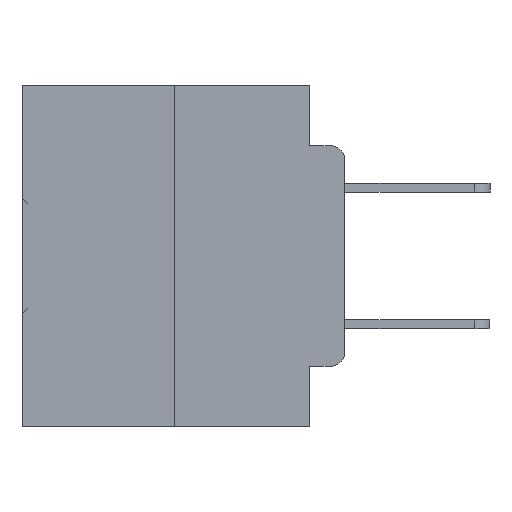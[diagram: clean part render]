
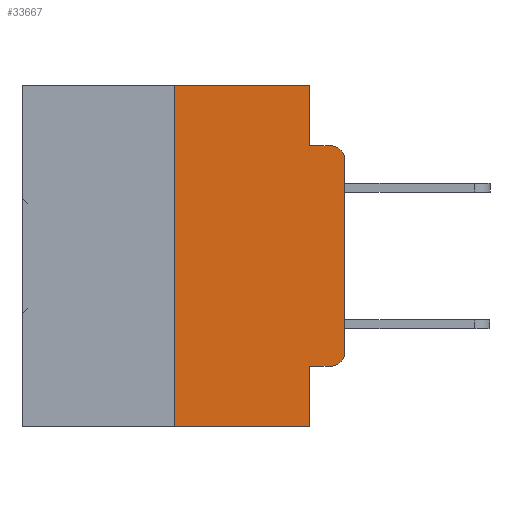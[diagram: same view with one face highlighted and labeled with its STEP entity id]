
A CAD part, left-side view. The second image highlights one B-rep face of the part: STEP entity #33667.
In plain terms, the highlighted planar face has unit normal (-1, 0, 0).
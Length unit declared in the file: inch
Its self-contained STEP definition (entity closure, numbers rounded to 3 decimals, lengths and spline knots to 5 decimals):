
#145 = EDGE_CURVE ( 'NONE', #18200, #20704, #22576, .T. ) ;
#853 = DIRECTION ( 'NONE',  ( 0., -1., 0. ) ) ;
#1075 = DIRECTION ( 'NONE',  ( 0., 0., -1. ) ) ;
#1307 = VERTEX_POINT ( 'NONE', #23346 ) ;
#1445 = CARTESIAN_POINT ( 'NONE',  ( 0., 0.051, 0. ) ) ;
#1585 = DIRECTION ( 'NONE',  ( 0., 0., -1. ) ) ;
#1717 = ORIENTED_EDGE ( 'NONE', *, *, #8641, .T. ) ;
#2132 = EDGE_CURVE ( 'NONE', #2736, #20704, #12573, .T. ) ;
#2736 = VERTEX_POINT ( 'NONE', #16717 ) ;
#3156 = DIRECTION ( 'NONE',  ( -1., 0., 0. ) ) ;
#4194 = DIRECTION ( 'NONE',  ( 0., -1., 0. ) ) ;
#4334 = ORIENTED_EDGE ( 'NONE', *, *, #32580, .T. ) ;
#4519 = PLANE ( 'NONE',  #10780 ) ;
#4811 = EDGE_CURVE ( 'NONE', #11716, #18200, #18731, .T. ) ;
#5305 = VERTEX_POINT ( 'NONE', #17956 ) ;
#5535 = VERTEX_POINT ( 'NONE', #29297 ) ;
#5775 = VECTOR ( 'NONE', #8782, 39.37008 ) ;
#7265 = CARTESIAN_POINT ( 'NONE',  ( 0., 0.473, 0. ) ) ;
#7304 = VERTEX_POINT ( 'NONE', #12982 ) ;
#7337 = LINE ( 'NONE', #9028, #33947 ) ;
#7715 = ORIENTED_EDGE ( 'NONE', *, *, #4811, .T. ) ;
#7801 = CARTESIAN_POINT ( 'NONE',  ( 0., 0.02, -0.4115 ) ) ;
#7810 = ORIENTED_EDGE ( 'NONE', *, *, #27281, .F. ) ;
#8641 = EDGE_CURVE ( 'NONE', #1307, #5305, #13774, .T. ) ;
#8782 = DIRECTION ( 'NONE',  ( 0., -1., 0. ) ) ;
#9028 = CARTESIAN_POINT ( 'NONE',  ( 0., 0.473, 0. ) ) ;
#9862 = AXIS2_PLACEMENT_3D ( 'NONE', #19339, #3156, #22029 ) ;
#10780 = AXIS2_PLACEMENT_3D ( 'NONE', #7265, #12646, #31262 ) ;
#11015 = AXIS2_PLACEMENT_3D ( 'NONE', #27876, #27852, #1075 ) ;
#11169 = CARTESIAN_POINT ( 'NONE',  ( 0., 0., -0.3915 ) ) ;
#11379 = CARTESIAN_POINT ( 'NONE',  ( 0., 0.25, 0. ) ) ;
#11716 = VERTEX_POINT ( 'NONE', #11169 ) ;
#11877 = VECTOR ( 'NONE', #853, 39.37008 ) ;
#12272 = EDGE_CURVE ( 'NONE', #1307, #7304, #22012, .T. ) ;
#12573 = LINE ( 'NONE', #17538, #26026 ) ;
#12646 = DIRECTION ( 'NONE',  ( 1., 0., 0. ) ) ;
#12814 = ORIENTED_EDGE ( 'NONE', *, *, #2132, .F. ) ;
#12982 = CARTESIAN_POINT ( 'NONE',  ( 0., 0.25, 0. ) ) ;
#13774 = LINE ( 'NONE', #27489, #5775 ) ;
#15287 = ORIENTED_EDGE ( 'NONE', *, *, #17733, .T. ) ;
#15960 = EDGE_LOOP ( 'NONE', ( #7715, #29438, #12814, #7810, #26127, #20745, #1717, #34269, #15287, #4334 ) ) ;
#16717 = CARTESIAN_POINT ( 'NONE',  ( 0., 0.051, -0.0885 ) ) ;
#17164 = DIRECTION ( 'NONE',  ( 0., -1., 0. ) ) ;
#17538 = CARTESIAN_POINT ( 'NONE',  ( 0., 0.051, -0.0885 ) ) ;
#17641 = DIRECTION ( 'NONE',  ( 0., 0., -1. ) ) ;
#17733 = EDGE_CURVE ( 'NONE', #26910, #34404, #19081, .T. ) ;
#17956 = CARTESIAN_POINT ( 'NONE',  ( 0., 0.051, -0.5 ) ) ;
#18200 = VERTEX_POINT ( 'NONE', #29771 ) ;
#18731 = LINE ( 'NONE', #21404, #26636 ) ;
#18932 = VECTOR ( 'NONE', #17641, 39.37008 ) ;
#19081 = LINE ( 'NONE', #19543, #11877 ) ;
#19339 = CARTESIAN_POINT ( 'NONE',  ( 0., 0.02, -0.3915 ) ) ;
#19543 = CARTESIAN_POINT ( 'NONE',  ( 0., 0.051, -0.4115 ) ) ;
#19749 = FACE_OUTER_BOUND ( 'NONE', #15960, .T. ) ;
#20349 = VECTOR ( 'NONE', #22112, 39.37008 ) ;
#20682 = EDGE_CURVE ( 'NONE', #26910, #5305, #34568, .T. ) ;
#20704 = VERTEX_POINT ( 'NONE', #31043 ) ;
#20745 = ORIENTED_EDGE ( 'NONE', *, *, #12272, .F. ) ;
#21404 = CARTESIAN_POINT ( 'NONE',  ( 0., 0., 0. ) ) ;
#21786 = CARTESIAN_POINT ( 'NONE',  ( 0., 0.051, -0.4115 ) ) ;
#22012 = LINE ( 'NONE', #11379, #20349 ) ;
#22029 = DIRECTION ( 'NONE',  ( 0., 0., -1. ) ) ;
#22112 = DIRECTION ( 'NONE',  ( 0., 0., 1. ) ) ;
#22388 = VECTOR ( 'NONE', #1585, 39.37008 ) ;
#22576 = CIRCLE ( 'NONE', #11015, 0.02 ) ;
#23346 = CARTESIAN_POINT ( 'NONE',  ( 0., 0.25, -0.5 ) ) ;
#24081 = DIRECTION ( 'NONE',  ( 0., 0., 1. ) ) ;
#26026 = VECTOR ( 'NONE', #4194, 39.37008 ) ;
#26127 = ORIENTED_EDGE ( 'NONE', *, *, #31500, .F. ) ;
#26636 = VECTOR ( 'NONE', #24081, 39.37008 ) ;
#26827 = CIRCLE ( 'NONE', #9862, 0.02 ) ;
#26910 = VERTEX_POINT ( 'NONE', #21786 ) ;
#27281 = EDGE_CURVE ( 'NONE', #5535, #2736, #29368, .T. ) ;
#27489 = CARTESIAN_POINT ( 'NONE',  ( 0., 0.473, -0.5 ) ) ;
#27852 = DIRECTION ( 'NONE',  ( -1., 0., 0. ) ) ;
#27876 = CARTESIAN_POINT ( 'NONE',  ( 0., 0.02, -0.1085 ) ) ;
#29297 = CARTESIAN_POINT ( 'NONE',  ( 0., 0.051, 0. ) ) ;
#29368 = LINE ( 'NONE', #33561, #22388 ) ;
#29438 = ORIENTED_EDGE ( 'NONE', *, *, #145, .T. ) ;
#29771 = CARTESIAN_POINT ( 'NONE',  ( 0., 0., -0.1085 ) ) ;
#31043 = CARTESIAN_POINT ( 'NONE',  ( 0., 0.02, -0.0885 ) ) ;
#31262 = DIRECTION ( 'NONE',  ( 0., 0., -1. ) ) ;
#31500 = EDGE_CURVE ( 'NONE', #7304, #5535, #7337, .T. ) ;
#32580 = EDGE_CURVE ( 'NONE', #34404, #11716, #26827, .T. ) ;
#33561 = CARTESIAN_POINT ( 'NONE',  ( 0., 0.051, 0. ) ) ;
#33667 = ADVANCED_FACE ( 'NONE', ( #19749 ), #4519, .F. ) ;
#33947 = VECTOR ( 'NONE', #17164, 39.37008 ) ;
#34269 = ORIENTED_EDGE ( 'NONE', *, *, #20682, .F. ) ;
#34404 = VERTEX_POINT ( 'NONE', #7801 ) ;
#34568 = LINE ( 'NONE', #1445, #18932 ) ;
